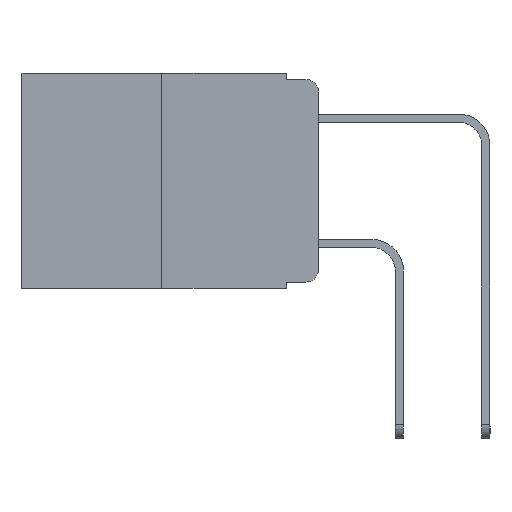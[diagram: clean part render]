
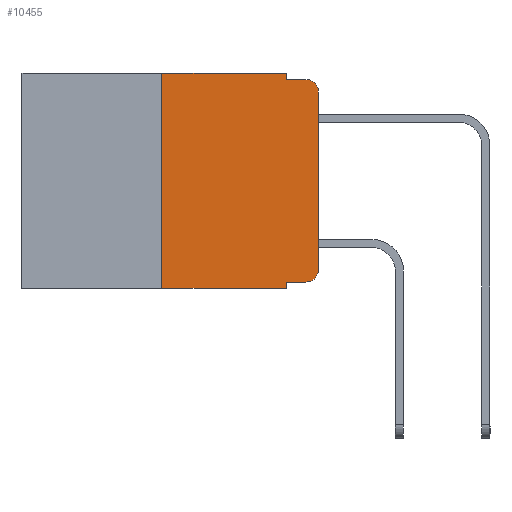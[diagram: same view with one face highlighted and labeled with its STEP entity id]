
A CAD part, left-side view. The second image highlights one B-rep face of the part: STEP entity #10455.
In plain terms, the highlighted planar face has unit normal (-1, 0, 0).
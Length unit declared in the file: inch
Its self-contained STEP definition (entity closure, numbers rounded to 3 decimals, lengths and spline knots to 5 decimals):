
#152 = VERTEX_POINT ( 'NONE', #13024 ) ;
#397 = EDGE_CURVE ( 'NONE', #152, #2604, #9496, .T. ) ;
#736 = CARTESIAN_POINT ( 'NONE',  ( 0., 0.051, 0. ) ) ;
#872 = CARTESIAN_POINT ( 'NONE',  ( 0., 0., 0. ) ) ;
#1195 = EDGE_CURVE ( 'NONE', #11861, #8755, #14096, .T. ) ;
#1642 = ORIENTED_EDGE ( 'NONE', *, *, #1195, .T. ) ;
#1659 = DIRECTION ( 'NONE',  ( 0., -1., 0. ) ) ;
#1848 = DIRECTION ( 'NONE',  ( 0., -1., 0. ) ) ;
#1874 = VECTOR ( 'NONE', #9669, 39.37008 ) ;
#1922 = ORIENTED_EDGE ( 'NONE', *, *, #6353, .T. ) ;
#1987 = ORIENTED_EDGE ( 'NONE', *, *, #5519, .T. ) ;
#2592 = LINE ( 'NONE', #4898, #5022 ) ;
#2604 = VERTEX_POINT ( 'NONE', #13809 ) ;
#2850 = CARTESIAN_POINT ( 'NONE',  ( 0., 0.25, 0. ) ) ;
#2927 = CARTESIAN_POINT ( 'NONE',  ( 0., 0.051, -0.01 ) ) ;
#3767 = VERTEX_POINT ( 'NONE', #736 ) ;
#4138 = FACE_OUTER_BOUND ( 'NONE', #5323, .T. ) ;
#4199 = LINE ( 'NONE', #7816, #10641 ) ;
#4205 = VERTEX_POINT ( 'NONE', #8883 ) ;
#4281 = CARTESIAN_POINT ( 'NONE',  ( 0., 0.25, -0.343 ) ) ;
#4308 = ORIENTED_EDGE ( 'NONE', *, *, #9292, .F. ) ;
#4807 = ORIENTED_EDGE ( 'NONE', *, *, #9990, .F. ) ;
#4850 = ORIENTED_EDGE ( 'NONE', *, *, #12584, .F. ) ;
#4898 = CARTESIAN_POINT ( 'NONE',  ( 0., 0.051, 0. ) ) ;
#5022 = VECTOR ( 'NONE', #13900, 39.37008 ) ;
#5218 = VERTEX_POINT ( 'NONE', #10113 ) ;
#5247 = PLANE ( 'NONE',  #13829 ) ;
#5285 = VERTEX_POINT ( 'NONE', #4281 ) ;
#5294 = VERTEX_POINT ( 'NONE', #8790 ) ;
#5323 = EDGE_LOOP ( 'NONE', ( #1987, #1642, #6394, #4807, #4308, #9565, #1922, #4850, #12024, #7297 ) ) ;
#5519 = EDGE_CURVE ( 'NONE', #6513, #11861, #10818, .T. ) ;
#5770 = DIRECTION ( 'NONE',  ( -1., 0., 0. ) ) ;
#6353 = EDGE_CURVE ( 'NONE', #5285, #5218, #7383, .T. ) ;
#6394 = ORIENTED_EDGE ( 'NONE', *, *, #13486, .F. ) ;
#6503 = DIRECTION ( 'NONE',  ( 0., 0., 1. ) ) ;
#6513 = VERTEX_POINT ( 'NONE', #6800 ) ;
#6800 = CARTESIAN_POINT ( 'NONE',  ( 0., 0., -0.313 ) ) ;
#6821 = VECTOR ( 'NONE', #11727, 39.37008 ) ;
#6881 = CARTESIAN_POINT ( 'NONE',  ( 0., 0.473, 0. ) ) ;
#7201 = CARTESIAN_POINT ( 'NONE',  ( 0., 0.051, 0. ) ) ;
#7297 = ORIENTED_EDGE ( 'NONE', *, *, #11062, .T. ) ;
#7383 = LINE ( 'NONE', #11920, #1874 ) ;
#7816 = CARTESIAN_POINT ( 'NONE',  ( 0., 0.473, 0. ) ) ;
#8234 = LINE ( 'NONE', #7201, #6821 ) ;
#8567 = VECTOR ( 'NONE', #6503, 39.37008 ) ;
#8688 = CARTESIAN_POINT ( 'NONE',  ( 0., 0.02, -0.01 ) ) ;
#8755 = VERTEX_POINT ( 'NONE', #8688 ) ;
#8790 = CARTESIAN_POINT ( 'NONE',  ( 0., 0.051, -0.01 ) ) ;
#8843 = VECTOR ( 'NONE', #1848, 39.37008 ) ;
#8883 = CARTESIAN_POINT ( 'NONE',  ( 0., 0.25, 0. ) ) ;
#9099 = DIRECTION ( 'NONE',  ( 0., 0., -1. ) ) ;
#9275 = CARTESIAN_POINT ( 'NONE',  ( 0., 0.02, -0.313 ) ) ;
#9292 = EDGE_CURVE ( 'NONE', #4205, #3767, #4199, .T. ) ;
#9496 = LINE ( 'NONE', #10902, #8843 ) ;
#9565 = ORIENTED_EDGE ( 'NONE', *, *, #12125, .F. ) ;
#9669 = DIRECTION ( 'NONE',  ( 0., -1., 0. ) ) ;
#9756 = CIRCLE ( 'NONE', #11193, 0.02 ) ;
#9990 = EDGE_CURVE ( 'NONE', #3767, #5294, #8234, .T. ) ;
#10113 = CARTESIAN_POINT ( 'NONE',  ( 0., 0.051, -0.343 ) ) ;
#10162 = DIRECTION ( 'NONE',  ( -1., 0., 0. ) ) ;
#10381 = VECTOR ( 'NONE', #13373, 39.37008 ) ;
#10455 = ADVANCED_FACE ( 'NONE', ( #4138 ), #5247, .F. ) ;
#10641 = VECTOR ( 'NONE', #12286, 39.37008 ) ;
#10818 = LINE ( 'NONE', #872, #10381 ) ;
#10902 = CARTESIAN_POINT ( 'NONE',  ( 0., 0.051, -0.333 ) ) ;
#11017 = AXIS2_PLACEMENT_3D ( 'NONE', #11400, #5770, #9099 ) ;
#11062 = EDGE_CURVE ( 'NONE', #2604, #6513, #9756, .T. ) ;
#11193 = AXIS2_PLACEMENT_3D ( 'NONE', #9275, #10162, #12636 ) ;
#11400 = CARTESIAN_POINT ( 'NONE',  ( 0., 0.02, -0.03 ) ) ;
#11727 = DIRECTION ( 'NONE',  ( 0., 0., -1. ) ) ;
#11846 = LINE ( 'NONE', #2927, #12887 ) ;
#11861 = VERTEX_POINT ( 'NONE', #14695 ) ;
#11920 = CARTESIAN_POINT ( 'NONE',  ( 0., 0.473, -0.343 ) ) ;
#12024 = ORIENTED_EDGE ( 'NONE', *, *, #397, .T. ) ;
#12125 = EDGE_CURVE ( 'NONE', #5285, #4205, #12138, .T. ) ;
#12138 = LINE ( 'NONE', #2850, #8567 ) ;
#12235 = DIRECTION ( 'NONE',  ( 0., 0., -1. ) ) ;
#12286 = DIRECTION ( 'NONE',  ( 0., -1., 0. ) ) ;
#12584 = EDGE_CURVE ( 'NONE', #152, #5218, #2592, .T. ) ;
#12636 = DIRECTION ( 'NONE',  ( 0., 0., -1. ) ) ;
#12887 = VECTOR ( 'NONE', #1659, 39.37008 ) ;
#13024 = CARTESIAN_POINT ( 'NONE',  ( 0., 0.051, -0.333 ) ) ;
#13373 = DIRECTION ( 'NONE',  ( 0., 0., 1. ) ) ;
#13486 = EDGE_CURVE ( 'NONE', #5294, #8755, #11846, .T. ) ;
#13569 = DIRECTION ( 'NONE',  ( 1., 0., 0. ) ) ;
#13809 = CARTESIAN_POINT ( 'NONE',  ( 0., 0.02, -0.333 ) ) ;
#13829 = AXIS2_PLACEMENT_3D ( 'NONE', #6881, #13569, #12235 ) ;
#13900 = DIRECTION ( 'NONE',  ( 0., 0., -1. ) ) ;
#14096 = CIRCLE ( 'NONE', #11017, 0.02 ) ;
#14695 = CARTESIAN_POINT ( 'NONE',  ( 0., 0., -0.03 ) ) ;
